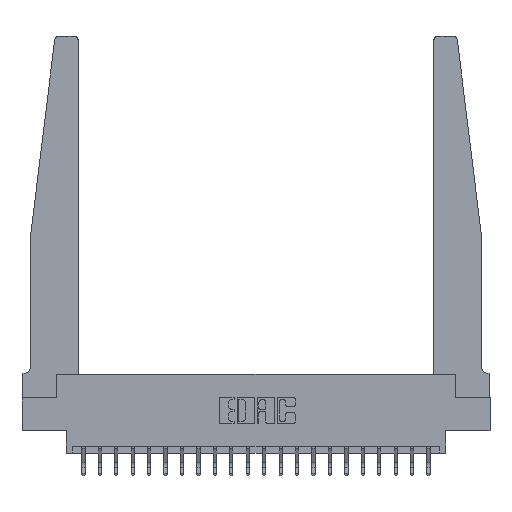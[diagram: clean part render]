
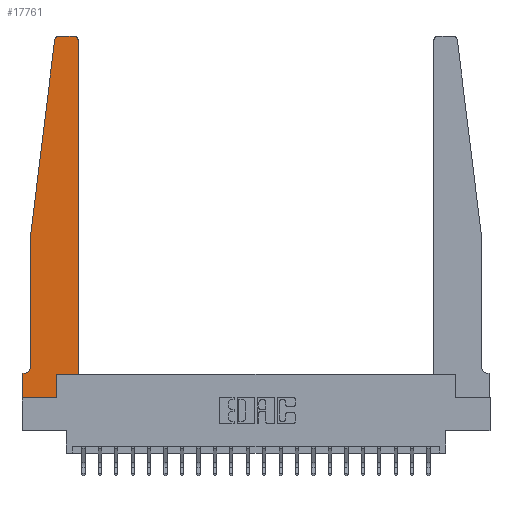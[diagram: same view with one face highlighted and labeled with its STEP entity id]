
A CAD part, top view. The second image highlights one B-rep face of the part: STEP entity #17761.
In plain terms, the highlighted planar face has unit normal (0, 0, 1).
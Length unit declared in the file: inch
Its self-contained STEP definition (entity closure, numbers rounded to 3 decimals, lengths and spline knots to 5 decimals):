
#167 = LINE ( 'NONE', #19420, #18683 ) ;
#204 = DIRECTION ( 'NONE',  ( -1., 0., 0. ) ) ;
#357 = ORIENTED_EDGE ( 'NONE', *, *, #1504, .T. ) ;
#516 = DIRECTION ( 'NONE',  ( 0., 0., 1. ) ) ;
#548 = ORIENTED_EDGE ( 'NONE', *, *, #4828, .T. ) ;
#978 = CARTESIAN_POINT ( 'NONE',  ( 0.425, 0.18, 0.37 ) ) ;
#1437 = AXIS2_PLACEMENT_3D ( 'NONE', #9952, #516, #11133 ) ;
#1504 = EDGE_CURVE ( 'NONE', #4087, #13598, #16443, .T. ) ;
#2181 = ORIENTED_EDGE ( 'NONE', *, *, #20050, .T. ) ;
#2182 = VECTOR ( 'NONE', #20776, 39.37008 ) ;
#2263 = EDGE_CURVE ( 'NONE', #9364, #12846, #6864, .T. ) ;
#2355 = CARTESIAN_POINT ( 'NONE',  ( 0.27653, 2.75, 0.37 ) ) ;
#2390 = EDGE_CURVE ( 'NONE', #12846, #4087, #12997, .T. ) ;
#2439 = CARTESIAN_POINT ( 'NONE',  ( 0.065, 1.25, 0.37 ) ) ;
#2580 = CARTESIAN_POINT ( 'NONE',  ( 0.065, 0.2375, 0.37 ) ) ;
#2657 = CARTESIAN_POINT ( 'NONE',  ( 0., 0.1875, 0.37 ) ) ;
#2669 = VECTOR ( 'NONE', #14542, 39.37008 ) ;
#2682 = DIRECTION ( 'NONE',  ( 0., 0., -1. ) ) ;
#2713 = DIRECTION ( 'NONE',  ( 0., 0., 1. ) ) ;
#3006 = ORIENTED_EDGE ( 'NONE', *, *, #4424, .T. ) ;
#3031 = DIRECTION ( 'NONE',  ( 1., 0., 0. ) ) ;
#3466 = DIRECTION ( 'NONE',  ( -0.122, -0.992, 0. ) ) ;
#3645 = EDGE_LOOP ( 'NONE', ( #19299, #19733, #3006, #548, #15495, #4778, #6132, #357, #14829, #12355, #10787, #2181 ) ) ;
#3705 = VERTEX_POINT ( 'NONE', #15536 ) ;
#4087 = VERTEX_POINT ( 'NONE', #20400 ) ;
#4424 = EDGE_CURVE ( 'NONE', #3705, #9426, #19184, .T. ) ;
#4778 = ORIENTED_EDGE ( 'NONE', *, *, #2263, .T. ) ;
#4828 = EDGE_CURVE ( 'NONE', #9426, #21604, #5580, .T. ) ;
#4995 = VERTEX_POINT ( 'NONE', #19055 ) ;
#5497 = VERTEX_POINT ( 'NONE', #12696 ) ;
#5580 = LINE ( 'NONE', #2439, #10251 ) ;
#5658 = EDGE_CURVE ( 'NONE', #13598, #4995, #167, .T. ) ;
#6034 = AXIS2_PLACEMENT_3D ( 'NONE', #22015, #2682, #15261 ) ;
#6132 = ORIENTED_EDGE ( 'NONE', *, *, #2390, .T. ) ;
#6864 = LINE ( 'NONE', #12115, #17545 ) ;
#7366 = CARTESIAN_POINT ( 'NONE',  ( 0.425, 0.18, 0.37 ) ) ;
#7844 = CARTESIAN_POINT ( 'NONE',  ( 0.2605, 0., 0.37 ) ) ;
#8883 = VECTOR ( 'NONE', #11823, 39.37008 ) ;
#9364 = VERTEX_POINT ( 'NONE', #10646 ) ;
#9426 = VERTEX_POINT ( 'NONE', #20949 ) ;
#9566 = DIRECTION ( 'NONE',  ( 0., -1., 0. ) ) ;
#9672 = CARTESIAN_POINT ( 'NONE',  ( 0., 0.1875, 0.37 ) ) ;
#9952 = CARTESIAN_POINT ( 'NONE',  ( 0.27653, 2.72, 0.37 ) ) ;
#10251 = VECTOR ( 'NONE', #19545, 39.37008 ) ;
#10387 = DIRECTION ( 'NONE',  ( -1., 0., 0. ) ) ;
#10646 = CARTESIAN_POINT ( 'NONE',  ( 0.015, 0.1875, 0.37 ) ) ;
#10787 = ORIENTED_EDGE ( 'NONE', *, *, #21697, .T. ) ;
#10874 = AXIS2_PLACEMENT_3D ( 'NONE', #16363, #2713, #14838 ) ;
#10941 = LINE ( 'NONE', #20911, #12728 ) ;
#11133 = DIRECTION ( 'NONE',  ( 1., 0., 0. ) ) ;
#11261 = CARTESIAN_POINT ( 'NONE',  ( 0., 0., 0.37 ) ) ;
#11306 = EDGE_CURVE ( 'NONE', #21604, #9364, #13304, .T. ) ;
#11723 = FACE_OUTER_BOUND ( 'NONE', #3645, .T. ) ;
#11823 = DIRECTION ( 'NONE',  ( 1., 0., 0. ) ) ;
#12115 = CARTESIAN_POINT ( 'NONE',  ( 0.065, 0.1875, 0.37 ) ) ;
#12355 = ORIENTED_EDGE ( 'NONE', *, *, #14431, .T. ) ;
#12696 = CARTESIAN_POINT ( 'NONE',  ( 0.425, 2.72, 0.37 ) ) ;
#12728 = VECTOR ( 'NONE', #204, 39.37008 ) ;
#12846 = VERTEX_POINT ( 'NONE', #2657 ) ;
#12997 = LINE ( 'NONE', #11261, #13129 ) ;
#13129 = VECTOR ( 'NONE', #9566, 39.37008 ) ;
#13165 = VECTOR ( 'NONE', #3466, 39.37008 ) ;
#13304 = CIRCLE ( 'NONE', #6034, 0.05 ) ;
#13315 = CARTESIAN_POINT ( 'NONE',  ( 0., 0., 0.37 ) ) ;
#13598 = VERTEX_POINT ( 'NONE', #7844 ) ;
#13616 = VERTEX_POINT ( 'NONE', #2355 ) ;
#13706 = VERTEX_POINT ( 'NONE', #978 ) ;
#13842 = CIRCLE ( 'NONE', #1437, 0.03 ) ;
#14339 = DIRECTION ( 'NONE',  ( 0., 1., 0. ) ) ;
#14431 = EDGE_CURVE ( 'NONE', #4995, #13706, #21204, .T. ) ;
#14542 = DIRECTION ( 'NONE',  ( 1., 0., 0. ) ) ;
#14555 = VERTEX_POINT ( 'NONE', #16129 ) ;
#14816 = LINE ( 'NONE', #21797, #2182 ) ;
#14829 = ORIENTED_EDGE ( 'NONE', *, *, #5658, .T. ) ;
#14838 = DIRECTION ( 'NONE',  ( 1., 0., 0. ) ) ;
#15261 = DIRECTION ( 'NONE',  ( -1., 0., 0. ) ) ;
#15495 = ORIENTED_EDGE ( 'NONE', *, *, #11306, .T. ) ;
#15536 = CARTESIAN_POINT ( 'NONE',  ( 0.24675, 2.72367, 0.37 ) ) ;
#16129 = CARTESIAN_POINT ( 'NONE',  ( 0.395, 2.75, 0.37 ) ) ;
#16363 = CARTESIAN_POINT ( 'NONE',  ( 0.395, 2.72, 0.37 ) ) ;
#16443 = LINE ( 'NONE', #13315, #8883 ) ;
#17107 = PLANE ( 'NONE',  #18405 ) ;
#17545 = VECTOR ( 'NONE', #10387, 39.37008 ) ;
#17761 = ADVANCED_FACE ( 'NONE', ( #11723 ), #17107, .T. ) ;
#18405 = AXIS2_PLACEMENT_3D ( 'NONE', #9672, #22257, #3031 ) ;
#18683 = VECTOR ( 'NONE', #14339, 39.37008 ) ;
#19055 = CARTESIAN_POINT ( 'NONE',  ( 0.2605, 0.18, 0.37 ) ) ;
#19184 = LINE ( 'NONE', #20871, #13165 ) ;
#19299 = ORIENTED_EDGE ( 'NONE', *, *, #20329, .T. ) ;
#19420 = CARTESIAN_POINT ( 'NONE',  ( 0.2605, 0.18, 0.37 ) ) ;
#19545 = DIRECTION ( 'NONE',  ( 0., -1., 0. ) ) ;
#19733 = ORIENTED_EDGE ( 'NONE', *, *, #20765, .T. ) ;
#20050 = EDGE_CURVE ( 'NONE', #5497, #14555, #20753, .T. ) ;
#20329 = EDGE_CURVE ( 'NONE', #14555, #13616, #10941, .T. ) ;
#20400 = CARTESIAN_POINT ( 'NONE',  ( 0., 0., 0.37 ) ) ;
#20753 = CIRCLE ( 'NONE', #10874, 0.03 ) ;
#20765 = EDGE_CURVE ( 'NONE', #13616, #3705, #13842, .T. ) ;
#20776 = DIRECTION ( 'NONE',  ( 0., 1., 0. ) ) ;
#20871 = CARTESIAN_POINT ( 'NONE',  ( 0.065, 1.25, 0.37 ) ) ;
#20911 = CARTESIAN_POINT ( 'NONE',  ( 0.25, 2.75, 0.37 ) ) ;
#20949 = CARTESIAN_POINT ( 'NONE',  ( 0.065, 1.25, 0.37 ) ) ;
#21204 = LINE ( 'NONE', #7366, #2669 ) ;
#21604 = VERTEX_POINT ( 'NONE', #2580 ) ;
#21697 = EDGE_CURVE ( 'NONE', #13706, #5497, #14816, .T. ) ;
#21797 = CARTESIAN_POINT ( 'NONE',  ( 0.425, 0.18, 0.37 ) ) ;
#22015 = CARTESIAN_POINT ( 'NONE',  ( 0.015, 0.2375, 0.37 ) ) ;
#22257 = DIRECTION ( 'NONE',  ( 0., 0., 1. ) ) ;
